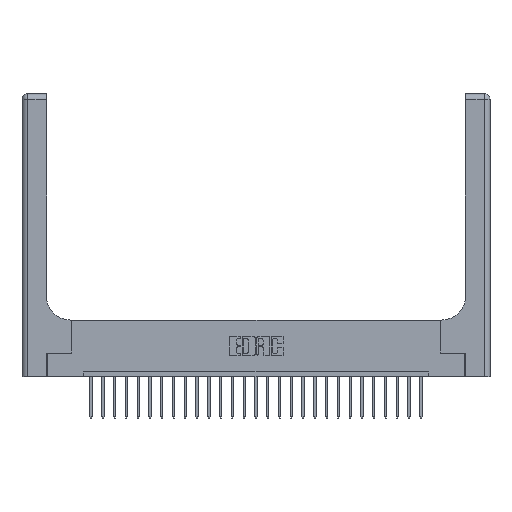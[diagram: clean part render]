
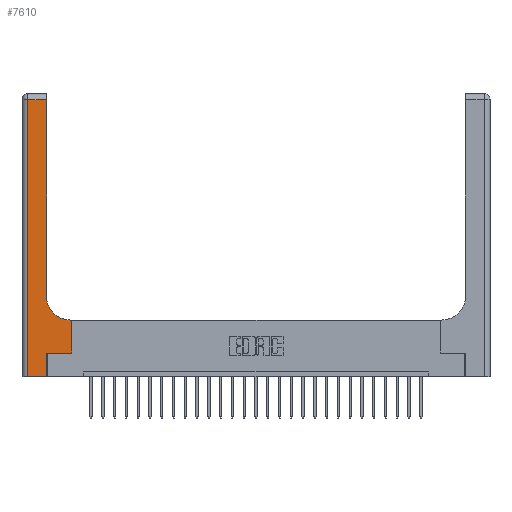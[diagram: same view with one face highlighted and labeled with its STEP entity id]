
A CAD part, top view. The second image highlights one B-rep face of the part: STEP entity #7610.
In plain terms, the highlighted planar face has unit normal (0, 0, 1).
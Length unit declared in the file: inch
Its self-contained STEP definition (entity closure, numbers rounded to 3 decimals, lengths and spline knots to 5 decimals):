
#172 = LINE ( 'NONE', #17901, #21852 ) ;
#485 = PLANE ( 'NONE',  #15841 ) ;
#1102 = ORIENTED_EDGE ( 'NONE', *, *, #14674, .T. ) ;
#1125 = DIRECTION ( 'NONE',  ( -1., 0., 0. ) ) ;
#1181 = VERTEX_POINT ( 'NONE', #6325 ) ;
#1665 = VERTEX_POINT ( 'NONE', #21170 ) ;
#1928 = VECTOR ( 'NONE', #15761, 39.37008 ) ;
#2413 = FACE_OUTER_BOUND ( 'NONE', #13514, .T. ) ;
#2475 = CARTESIAN_POINT ( 'NONE',  ( 0.265, 0.25, 0.37 ) ) ;
#2545 = LINE ( 'NONE', #16422, #19687 ) ;
#2675 = DIRECTION ( 'NONE',  ( 0., 0., -1. ) ) ;
#3438 = VERTEX_POINT ( 'NONE', #17663 ) ;
#3644 = VERTEX_POINT ( 'NONE', #13291 ) ;
#4458 = VECTOR ( 'NONE', #1125, 39.37008 ) ;
#5014 = VERTEX_POINT ( 'NONE', #9932 ) ;
#5288 = ORIENTED_EDGE ( 'NONE', *, *, #16288, .T. ) ;
#5461 = EDGE_CURVE ( 'NONE', #5014, #3438, #6084, .T. ) ;
#6084 = LINE ( 'NONE', #2475, #22305 ) ;
#6325 = CARTESIAN_POINT ( 'NONE',  ( 0.51, 0.6, 0.37 ) ) ;
#7610 = ADVANCED_FACE ( 'NONE', ( #2413 ), #485, .F. ) ;
#8142 = DIRECTION ( 'NONE',  ( 0., 1., 0. ) ) ;
#9114 = DIRECTION ( 'NONE',  ( 0., -1., 0. ) ) ;
#9918 = ORIENTED_EDGE ( 'NONE', *, *, #20035, .T. ) ;
#9932 = CARTESIAN_POINT ( 'NONE',  ( 0.265, 0.25, 0.37 ) ) ;
#10256 = DIRECTION ( 'NONE',  ( 0., 1., 0. ) ) ;
#10389 = DIRECTION ( 'NONE',  ( -1., 0., 0. ) ) ;
#10618 = CARTESIAN_POINT ( 'NONE',  ( 0.06, 2.94, 0.37 ) ) ;
#11643 = DIRECTION ( 'NONE',  ( 0., 0., -1. ) ) ;
#11658 = ORIENTED_EDGE ( 'NONE', *, *, #16712, .T. ) ;
#12409 = ORIENTED_EDGE ( 'NONE', *, *, #21257, .T. ) ;
#13291 = CARTESIAN_POINT ( 'NONE',  ( 0.265, 0., 0.37 ) ) ;
#13514 = EDGE_LOOP ( 'NONE', ( #11658, #9918, #1102, #21240, #12409, #14401, #18348, #5288, #14615 ) ) ;
#13682 = VECTOR ( 'NONE', #22287, 39.37008 ) ;
#14401 = ORIENTED_EDGE ( 'NONE', *, *, #5461, .T. ) ;
#14569 = VERTEX_POINT ( 'NONE', #15150 ) ;
#14615 = ORIENTED_EDGE ( 'NONE', *, *, #16308, .T. ) ;
#14646 = CARTESIAN_POINT ( 'NONE',  ( 0., 0., 0.37 ) ) ;
#14674 = EDGE_CURVE ( 'NONE', #22779, #15999, #25274, .T. ) ;
#15150 = CARTESIAN_POINT ( 'NONE',  ( 0.528, 0.6, 0.37 ) ) ;
#15761 = DIRECTION ( 'NONE',  ( -1., 0., 0. ) ) ;
#15841 = AXIS2_PLACEMENT_3D ( 'NONE', #20147, #2675, #10389 ) ;
#15999 = VERTEX_POINT ( 'NONE', #16161 ) ;
#16123 = LINE ( 'NONE', #23952, #13682 ) ;
#16161 = CARTESIAN_POINT ( 'NONE',  ( 0.06, 0., 0.37 ) ) ;
#16288 = EDGE_CURVE ( 'NONE', #14569, #1181, #19988, .T. ) ;
#16308 = EDGE_CURVE ( 'NONE', #1181, #17690, #21626, .T. ) ;
#16312 = VECTOR ( 'NONE', #9114, 39.37008 ) ;
#16422 = CARTESIAN_POINT ( 'NONE',  ( 0.265, 0., 0.37 ) ) ;
#16712 = EDGE_CURVE ( 'NONE', #17690, #1665, #172, .T. ) ;
#17408 = VECTOR ( 'NONE', #21056, 39.37008 ) ;
#17558 = EDGE_CURVE ( 'NONE', #3438, #14569, #16123, .T. ) ;
#17663 = CARTESIAN_POINT ( 'NONE',  ( 0.528, 0.25, 0.37 ) ) ;
#17690 = VERTEX_POINT ( 'NONE', #20863 ) ;
#17901 = CARTESIAN_POINT ( 'NONE',  ( 0.26, 3., 0.37 ) ) ;
#18348 = ORIENTED_EDGE ( 'NONE', *, *, #17558, .T. ) ;
#18384 = EDGE_CURVE ( 'NONE', #15999, #3644, #22472, .T. ) ;
#18874 = CARTESIAN_POINT ( 'NONE',  ( 0.06, 3., 0.37 ) ) ;
#18982 = LINE ( 'NONE', #22571, #4458 ) ;
#19687 = VECTOR ( 'NONE', #10256, 39.37008 ) ;
#19988 = LINE ( 'NONE', #23581, #1928 ) ;
#20035 = EDGE_CURVE ( 'NONE', #1665, #22779, #18982, .T. ) ;
#20147 = CARTESIAN_POINT ( 'NONE',  ( 0., 3., 0.37 ) ) ;
#20340 = DIRECTION ( 'NONE',  ( 1., 0., 0. ) ) ;
#20863 = CARTESIAN_POINT ( 'NONE',  ( 0.26, 0.85, 0.37 ) ) ;
#21056 = DIRECTION ( 'NONE',  ( 1., 0., 0. ) ) ;
#21170 = CARTESIAN_POINT ( 'NONE',  ( 0.26, 2.94, 0.37 ) ) ;
#21240 = ORIENTED_EDGE ( 'NONE', *, *, #18384, .T. ) ;
#21257 = EDGE_CURVE ( 'NONE', #3644, #5014, #2545, .T. ) ;
#21626 = CIRCLE ( 'NONE', #23673, 0.25 ) ;
#21852 = VECTOR ( 'NONE', #8142, 39.37008 ) ;
#21912 = DIRECTION ( 'NONE',  ( 1., 0., 0. ) ) ;
#22038 = CARTESIAN_POINT ( 'NONE',  ( 0.51, 0.85, 0.37 ) ) ;
#22287 = DIRECTION ( 'NONE',  ( 0., 1., 0. ) ) ;
#22305 = VECTOR ( 'NONE', #20340, 39.37008 ) ;
#22472 = LINE ( 'NONE', #14646, #17408 ) ;
#22571 = CARTESIAN_POINT ( 'NONE',  ( 0., 2.94, 0.37 ) ) ;
#22779 = VERTEX_POINT ( 'NONE', #10618 ) ;
#23581 = CARTESIAN_POINT ( 'NONE',  ( 0.26, 0.6, 0.37 ) ) ;
#23673 = AXIS2_PLACEMENT_3D ( 'NONE', #22038, #11643, #21912 ) ;
#23952 = CARTESIAN_POINT ( 'NONE',  ( 0.528, 0.25, 0.37 ) ) ;
#25274 = LINE ( 'NONE', #18874, #16312 ) ;
